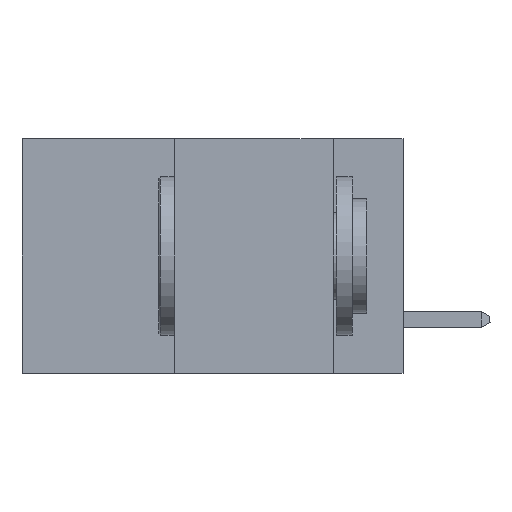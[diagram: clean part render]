
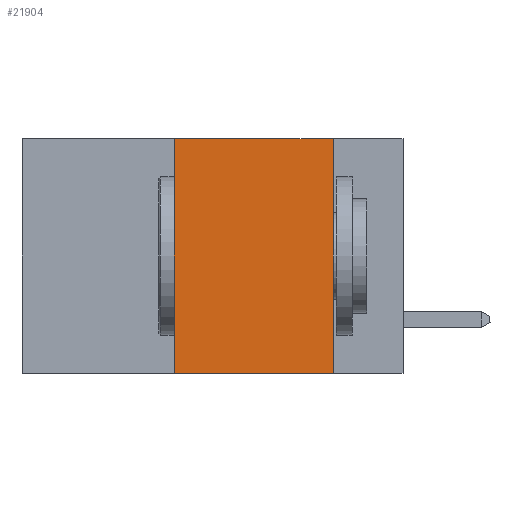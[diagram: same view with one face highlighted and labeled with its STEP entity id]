
A CAD part, left-side view. The second image highlights one B-rep face of the part: STEP entity #21904.
In plain terms, the highlighted planar face has unit normal (-1, 0, 0).
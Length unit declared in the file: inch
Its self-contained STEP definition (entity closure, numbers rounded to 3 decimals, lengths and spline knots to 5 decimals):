
#1126 = ORIENTED_EDGE ( 'NONE', *, *, #37523, .F. ) ;
#2163 = CARTESIAN_POINT ( 'NONE',  ( 0., 0.36, 0. ) ) ;
#3153 = DIRECTION ( 'NONE',  ( 1., 0., 0. ) ) ;
#4018 = EDGE_CURVE ( 'NONE', #11243, #29777, #48520, .T. ) ;
#4757 = VECTOR ( 'NONE', #35969, 39.37008 ) ;
#4997 = CARTESIAN_POINT ( 'NONE',  ( 0., 0.36, 0. ) ) ;
#7546 = EDGE_LOOP ( 'NONE', ( #40791, #46886, #1126, #39749 ) ) ;
#7988 = LINE ( 'NONE', #30811, #35327 ) ;
#8316 = VECTOR ( 'NONE', #25435, 39.37008 ) ;
#11243 = VERTEX_POINT ( 'NONE', #49390 ) ;
#11885 = CARTESIAN_POINT ( 'NONE',  ( 0., 0.11, -0.37 ) ) ;
#13093 = CARTESIAN_POINT ( 'NONE',  ( 0., 0.11, 0. ) ) ;
#13303 = VECTOR ( 'NONE', #13956, 39.37008 ) ;
#13956 = DIRECTION ( 'NONE',  ( 0., -1., 0. ) ) ;
#18412 = VERTEX_POINT ( 'NONE', #26161 ) ;
#20920 = EDGE_CURVE ( 'NONE', #18412, #29777, #7988, .T. ) ;
#21904 = ADVANCED_FACE ( 'NONE', ( #40697 ), #22331, .F. ) ;
#22331 = PLANE ( 'NONE',  #50161 ) ;
#24222 = LINE ( 'NONE', #29870, #13303 ) ;
#25435 = DIRECTION ( 'NONE',  ( 0., 0., 1. ) ) ;
#26161 = CARTESIAN_POINT ( 'NONE',  ( 0., 0.36, -0.37 ) ) ;
#26267 = CARTESIAN_POINT ( 'NONE',  ( 0., 0.6, 0. ) ) ;
#29777 = VERTEX_POINT ( 'NONE', #11885 ) ;
#29870 = CARTESIAN_POINT ( 'NONE',  ( 0., 0.6, 0. ) ) ;
#30811 = CARTESIAN_POINT ( 'NONE',  ( 0., 0.6, -0.37 ) ) ;
#33848 = LINE ( 'NONE', #2163, #8316 ) ;
#34211 = EDGE_CURVE ( 'NONE', #42930, #11243, #24222, .T. ) ;
#35327 = VECTOR ( 'NONE', #46415, 39.37008 ) ;
#35969 = DIRECTION ( 'NONE',  ( 0., 0., -1. ) ) ;
#37523 = EDGE_CURVE ( 'NONE', #18412, #42930, #33848, .T. ) ;
#39749 = ORIENTED_EDGE ( 'NONE', *, *, #20920, .T. ) ;
#40697 = FACE_OUTER_BOUND ( 'NONE', #7546, .T. ) ;
#40791 = ORIENTED_EDGE ( 'NONE', *, *, #4018, .F. ) ;
#42930 = VERTEX_POINT ( 'NONE', #4997 ) ;
#46415 = DIRECTION ( 'NONE',  ( 0., -1., 0. ) ) ;
#46886 = ORIENTED_EDGE ( 'NONE', *, *, #34211, .F. ) ;
#47112 = DIRECTION ( 'NONE',  ( 0., 0., -1. ) ) ;
#48520 = LINE ( 'NONE', #13093, #4757 ) ;
#49390 = CARTESIAN_POINT ( 'NONE',  ( 0., 0.11, 0. ) ) ;
#50161 = AXIS2_PLACEMENT_3D ( 'NONE', #26267, #3153, #47112 ) ;
